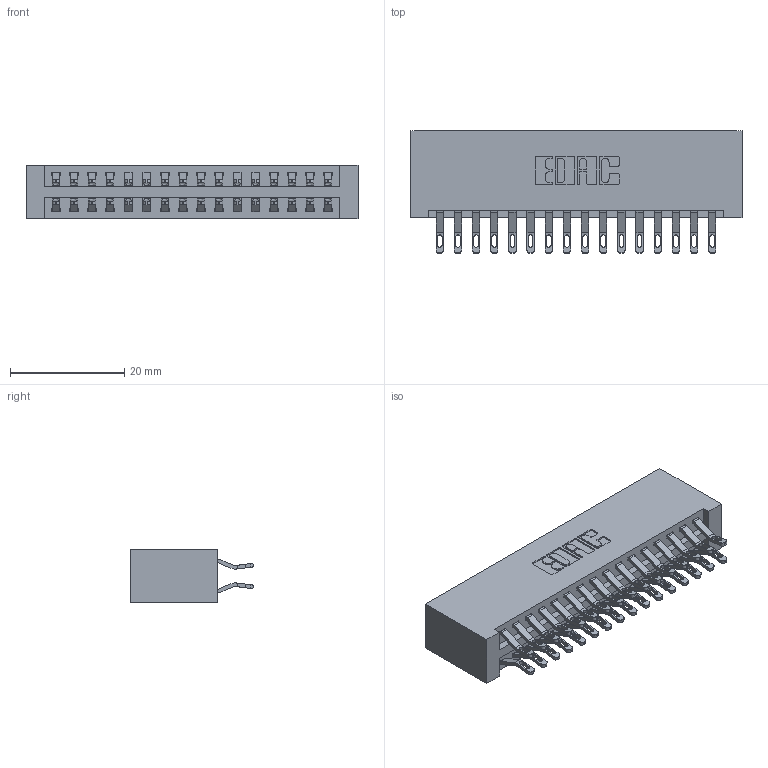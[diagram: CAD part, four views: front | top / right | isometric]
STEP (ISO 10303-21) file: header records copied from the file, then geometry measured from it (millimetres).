
FILE_DESCRIPTION (( 'STEP AP203' ), '1' );
FILE_NAME ('396-032-555-201.STEP', '2018-09-05T11:25:43', ( '' ), ( '' ), 'SwSTEP 2.0', 'SolidWorks 2016', '' );
FILE_SCHEMA (( 'CONFIG_CONTROL_DESIGN' ));
Length unit declared in the file: inch
Products named in the file (3): 346 Part_No Mounting Lugs; 345-292-001_555 Tail; 396-032-555-201
Assembly tree (33 placements, depth 2):
  396-032-555-201
    346 Part_No Mounting Lugs
    345-292-001_555 Tail  x32
Bounding box: 58.04 x 21.46 x 9.4 mm (x, y, z)
Volume: 6123.7 mm3; surface area: 8502.8 mm2
Topology: 33 solids, 33 shells, 1970 faces, 6161 edges, 4106 vertices
Faces by surface type: plane 1128, cylinder 842
Entity records: 13991 total; most frequent: CARTESIAN_POINT 2374, ORIENTED_EDGE 2278, DIRECTION 2107, EDGE_CURVE 1139, LINE 931, VECTOR 931, VERTEX_POINT 758, AXIS2_PLACEMENT_3D 588
